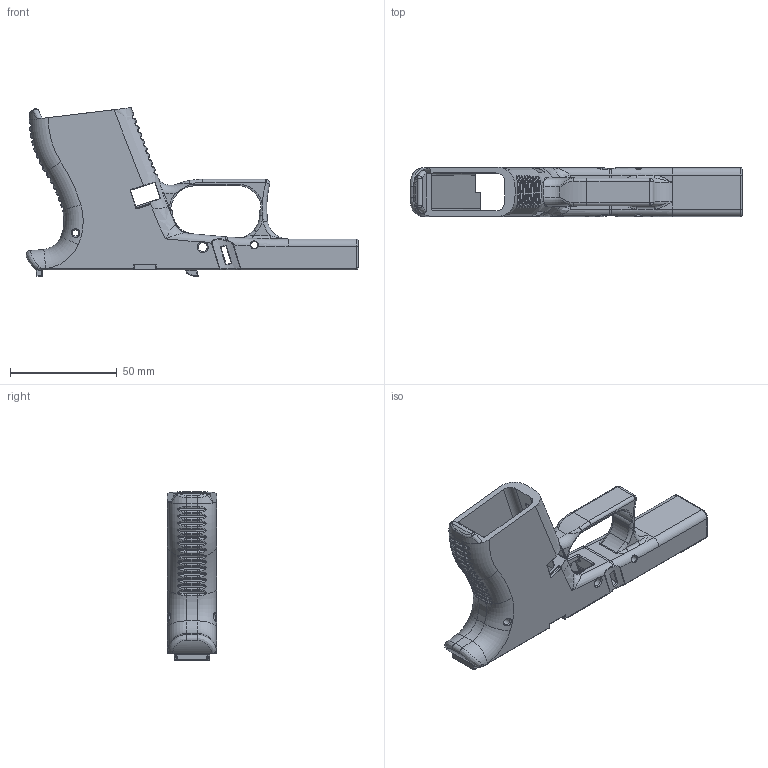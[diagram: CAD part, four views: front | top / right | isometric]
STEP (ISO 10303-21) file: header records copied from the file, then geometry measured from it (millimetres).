
FILE_DESCRIPTION(/* description */ (''),/* implementation_level */ '2;1');
FILE_NAME(/* name */ 'Frame.step',/* time_stamp */ '2021-12-05T09:29:05-05:00',/* author */ (''),/* organization */ (''),/* preprocessor_version */ 'ST-DEVELOPER v18.1',/* originating_system */ 'Autodesk Translation Framework v10.10.0.1391',/* authorisation */ '');
FILE_SCHEMA (('AUTOMOTIVE_DESIGN { 1 0 10303 214 3 1 1 }'));
Products named in the file (2): Frame; Rails and Internals
Assembly tree (1 placements, depth 2):
  Frame
    Rails and Internals
Bounding box: 155.83 x 23 x 79.14 mm (x, y, z)
Volume: 48231.2 mm3; surface area: 31952.2 mm2
Topology: 1 solids, 1 shells, 1268 faces, 3174 edges, 1849 vertices
Faces by surface type: bspline 510, cylinder 380, plane 227, torus 100, sphere 30, cone 21
Full cylindrical faces by diameter (mm): 3.05 x2, 3.3 x2, 3.5 x1, 4.25 x2
Entity records: 54006 total; most frequent: CARTESIAN_POINT 25817, ORIENTED_EDGE 6264, DIRECTION 5465, EDGE_CURVE 3132, AXIS2_PLACEMENT_3D 2226, VERTEX_POINT 1849, EDGE_LOOP 1277, FACE_OUTER_BOUND 1268
